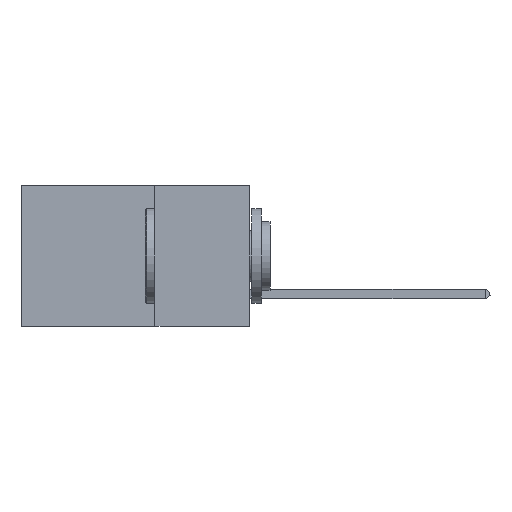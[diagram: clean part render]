
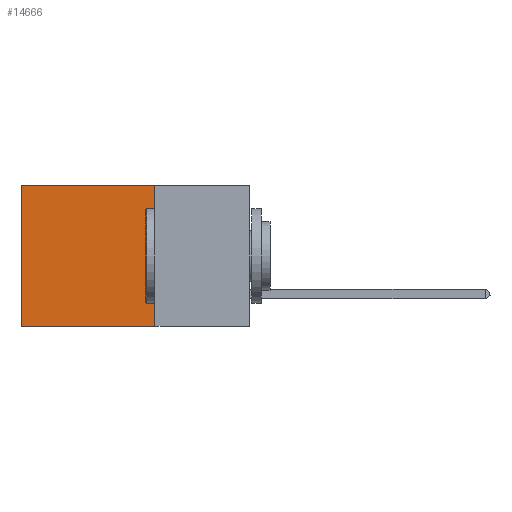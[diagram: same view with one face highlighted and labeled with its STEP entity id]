
A CAD part, left-side view. The second image highlights one B-rep face of the part: STEP entity #14666.
In plain terms, the highlighted planar face has unit normal (-1, 0, 0).
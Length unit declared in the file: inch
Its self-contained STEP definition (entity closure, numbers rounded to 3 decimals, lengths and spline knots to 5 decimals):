
#1071 = VERTEX_POINT ( 'NONE', #17096 ) ;
#1428 = FACE_OUTER_BOUND ( 'NONE', #12796, .T. ) ;
#2402 = CARTESIAN_POINT ( 'NONE',  ( 0.2875, 0.25, 0. ) ) ;
#2551 = ORIENTED_EDGE ( 'NONE', *, *, #18710, .T. ) ;
#3272 = LINE ( 'NONE', #18096, #24120 ) ;
#4431 = DIRECTION ( 'NONE',  ( 1., 0., 0. ) ) ;
#5178 = CARTESIAN_POINT ( 'NONE',  ( 0.2875, 0.25, 0. ) ) ;
#5713 = EDGE_CURVE ( 'NONE', #1071, #15220, #7874, .T. ) ;
#7749 = CARTESIAN_POINT ( 'NONE',  ( 0.2875, 0.25, -0.37 ) ) ;
#7874 = LINE ( 'NONE', #7749, #22091 ) ;
#8755 = AXIS2_PLACEMENT_3D ( 'NONE', #2402, #4431, #17307 ) ;
#10002 = EDGE_CURVE ( 'NONE', #18723, #15220, #3272, .T. ) ;
#11348 = VERTEX_POINT ( 'NONE', #25847 ) ;
#12796 = EDGE_LOOP ( 'NONE', ( #23537, #19861, #22826, #2551 ) ) ;
#13083 = LINE ( 'NONE', #5178, #19708 ) ;
#13568 = LINE ( 'NONE', #21716, #17968 ) ;
#14455 = PLANE ( 'NONE',  #8755 ) ;
#14666 = ADVANCED_FACE ( 'NONE', ( #1428 ), #14455, .F. ) ;
#15220 = VERTEX_POINT ( 'NONE', #16449 ) ;
#16449 = CARTESIAN_POINT ( 'NONE',  ( 0.2875, 0.6, -0.37 ) ) ;
#17096 = CARTESIAN_POINT ( 'NONE',  ( 0.2875, 0.25, -0.37 ) ) ;
#17307 = DIRECTION ( 'NONE',  ( 0., 0., -1. ) ) ;
#17968 = VECTOR ( 'NONE', #25398, 39.37008 ) ;
#18096 = CARTESIAN_POINT ( 'NONE',  ( 0.2875, 0.6, 0. ) ) ;
#18710 = EDGE_CURVE ( 'NONE', #11348, #18723, #13083, .T. ) ;
#18723 = VERTEX_POINT ( 'NONE', #19198 ) ;
#19198 = CARTESIAN_POINT ( 'NONE',  ( 0.2875, 0.6, 0. ) ) ;
#19708 = VECTOR ( 'NONE', #24982, 39.37008 ) ;
#19861 = ORIENTED_EDGE ( 'NONE', *, *, #5713, .F. ) ;
#19992 = EDGE_CURVE ( 'NONE', #11348, #1071, #13568, .T. ) ;
#21716 = CARTESIAN_POINT ( 'NONE',  ( 0.2875, 0.25, 0. ) ) ;
#22091 = VECTOR ( 'NONE', #22146, 39.37008 ) ;
#22121 = DIRECTION ( 'NONE',  ( 0., 0., -1. ) ) ;
#22146 = DIRECTION ( 'NONE',  ( 0., 1., 0. ) ) ;
#22826 = ORIENTED_EDGE ( 'NONE', *, *, #19992, .F. ) ;
#23537 = ORIENTED_EDGE ( 'NONE', *, *, #10002, .T. ) ;
#24120 = VECTOR ( 'NONE', #22121, 39.37008 ) ;
#24982 = DIRECTION ( 'NONE',  ( 0., 1., 0. ) ) ;
#25398 = DIRECTION ( 'NONE',  ( 0., 0., -1. ) ) ;
#25847 = CARTESIAN_POINT ( 'NONE',  ( 0.2875, 0.25, 0. ) ) ;
